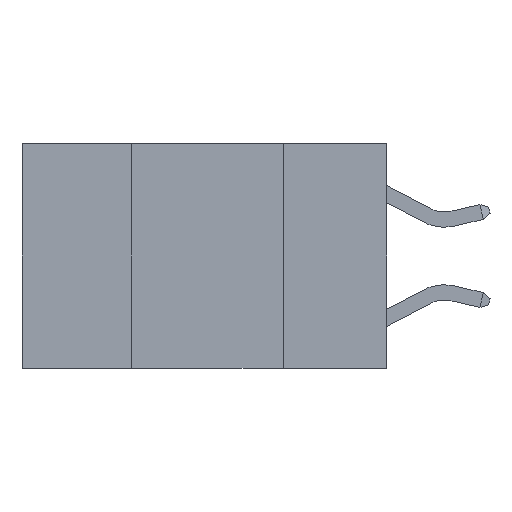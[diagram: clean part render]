
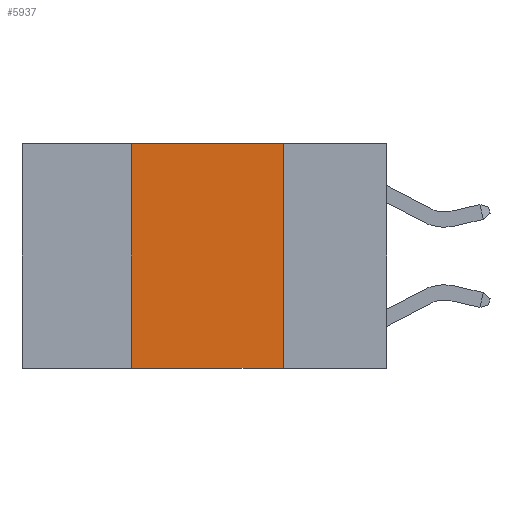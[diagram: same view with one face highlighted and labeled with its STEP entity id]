
A CAD part, left-side view. The second image highlights one B-rep face of the part: STEP entity #5937.
In plain terms, the highlighted planar face has unit normal (-1, 0, 0).
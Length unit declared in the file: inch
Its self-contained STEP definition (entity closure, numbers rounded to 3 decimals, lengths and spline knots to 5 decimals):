
#1678 = EDGE_CURVE ( 'NONE', #8666, #4758, #2236, .T. ) ;
#2087 = CARTESIAN_POINT ( 'NONE',  ( 0., 0.17, 0. ) ) ;
#2221 = CARTESIAN_POINT ( 'NONE',  ( 0., 0.17, -0.37 ) ) ;
#2236 = LINE ( 'NONE', #9917, #4354 ) ;
#2432 = ORIENTED_EDGE ( 'NONE', *, *, #4079, .F. ) ;
#2495 = CARTESIAN_POINT ( 'NONE',  ( 0., 0.6, 0. ) ) ;
#2671 = AXIS2_PLACEMENT_3D ( 'NONE', #10908, #9898, #8633 ) ;
#2679 = LINE ( 'NONE', #4628, #9595 ) ;
#2864 = EDGE_LOOP ( 'NONE', ( #13350, #2432, #12936, #13510 ) ) ;
#3367 = FACE_OUTER_BOUND ( 'NONE', #2864, .T. ) ;
#3578 = LINE ( 'NONE', #2495, #14186 ) ;
#4079 = EDGE_CURVE ( 'NONE', #4758, #11995, #3578, .T. ) ;
#4173 = PLANE ( 'NONE',  #2671 ) ;
#4354 = VECTOR ( 'NONE', #10930, 39.37008 ) ;
#4628 = CARTESIAN_POINT ( 'NONE',  ( 0., 0.6, -0.37 ) ) ;
#4676 = CARTESIAN_POINT ( 'NONE',  ( 0., 0.42, 0. ) ) ;
#4758 = VERTEX_POINT ( 'NONE', #4676 ) ;
#5937 = ADVANCED_FACE ( 'NONE', ( #3367 ), #4173, .F. ) ;
#8633 = DIRECTION ( 'NONE',  ( 0., 0., -1. ) ) ;
#8666 = VERTEX_POINT ( 'NONE', #13678 ) ;
#9106 = DIRECTION ( 'NONE',  ( 0., -1., 0. ) ) ;
#9595 = VECTOR ( 'NONE', #12521, 39.37008 ) ;
#9898 = DIRECTION ( 'NONE',  ( 1., 0., 0. ) ) ;
#9917 = CARTESIAN_POINT ( 'NONE',  ( 0., 0.42, 0. ) ) ;
#9978 = CARTESIAN_POINT ( 'NONE',  ( 0., 0.17, 0. ) ) ;
#10601 = EDGE_CURVE ( 'NONE', #11995, #12141, #12895, .T. ) ;
#10908 = CARTESIAN_POINT ( 'NONE',  ( 0., 0.6, 0. ) ) ;
#10930 = DIRECTION ( 'NONE',  ( 0., 0., 1. ) ) ;
#11074 = VECTOR ( 'NONE', #13955, 39.37008 ) ;
#11995 = VERTEX_POINT ( 'NONE', #9978 ) ;
#12141 = VERTEX_POINT ( 'NONE', #2221 ) ;
#12521 = DIRECTION ( 'NONE',  ( 0., -1., 0. ) ) ;
#12895 = LINE ( 'NONE', #2087, #11074 ) ;
#12936 = ORIENTED_EDGE ( 'NONE', *, *, #1678, .F. ) ;
#13350 = ORIENTED_EDGE ( 'NONE', *, *, #10601, .F. ) ;
#13510 = ORIENTED_EDGE ( 'NONE', *, *, #13544, .T. ) ;
#13544 = EDGE_CURVE ( 'NONE', #8666, #12141, #2679, .T. ) ;
#13678 = CARTESIAN_POINT ( 'NONE',  ( 0., 0.42, -0.37 ) ) ;
#13955 = DIRECTION ( 'NONE',  ( 0., 0., -1. ) ) ;
#14186 = VECTOR ( 'NONE', #9106, 39.37008 ) ;
